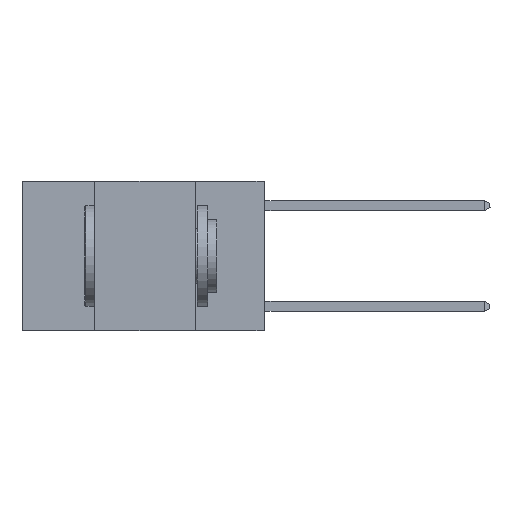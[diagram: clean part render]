
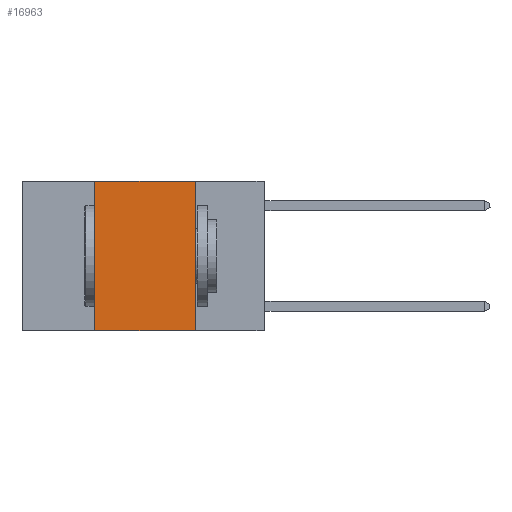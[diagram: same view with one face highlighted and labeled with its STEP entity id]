
A CAD part, left-side view. The second image highlights one B-rep face of the part: STEP entity #16963.
In plain terms, the highlighted planar face has unit normal (-1, 0, 0).
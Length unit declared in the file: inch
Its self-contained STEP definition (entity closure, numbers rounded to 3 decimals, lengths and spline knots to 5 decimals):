
#492 = CARTESIAN_POINT ( 'NONE',  ( 0., 0.42, 0. ) ) ;
#1504 = LINE ( 'NONE', #22077, #13023 ) ;
#2939 = VERTEX_POINT ( 'NONE', #27327 ) ;
#2967 = ORIENTED_EDGE ( 'NONE', *, *, #24986, .F. ) ;
#2998 = VECTOR ( 'NONE', #12646, 39.37008 ) ;
#4350 = PLANE ( 'NONE',  #23697 ) ;
#5289 = VERTEX_POINT ( 'NONE', #22720 ) ;
#6217 = LINE ( 'NONE', #11053, #22846 ) ;
#6974 = EDGE_CURVE ( 'NONE', #17826, #8032, #21175, .T. ) ;
#7304 = CARTESIAN_POINT ( 'NONE',  ( 0., 0.42, -0.37 ) ) ;
#8032 = VERTEX_POINT ( 'NONE', #492 ) ;
#8405 = ORIENTED_EDGE ( 'NONE', *, *, #6974, .F. ) ;
#8835 = DIRECTION ( 'NONE',  ( 0., -1., 0. ) ) ;
#9549 = CARTESIAN_POINT ( 'NONE',  ( 0., 0.17, 0. ) ) ;
#10318 = CARTESIAN_POINT ( 'NONE',  ( 0., 0.42, 0. ) ) ;
#11053 = CARTESIAN_POINT ( 'NONE',  ( 0., 0.6, 0. ) ) ;
#11268 = DIRECTION ( 'NONE',  ( 0., 0., -1. ) ) ;
#12646 = DIRECTION ( 'NONE',  ( 0., 0., 1. ) ) ;
#13023 = VECTOR ( 'NONE', #17570, 39.37008 ) ;
#13420 = EDGE_LOOP ( 'NONE', ( #14421, #2967, #8405, #14351 ) ) ;
#14351 = ORIENTED_EDGE ( 'NONE', *, *, #14888, .T. ) ;
#14421 = ORIENTED_EDGE ( 'NONE', *, *, #22596, .F. ) ;
#14888 = EDGE_CURVE ( 'NONE', #17826, #5289, #1504, .T. ) ;
#16352 = LINE ( 'NONE', #9549, #22328 ) ;
#16963 = ADVANCED_FACE ( 'NONE', ( #23442 ), #4350, .F. ) ;
#17570 = DIRECTION ( 'NONE',  ( 0., -1., 0. ) ) ;
#17826 = VERTEX_POINT ( 'NONE', #7304 ) ;
#20865 = DIRECTION ( 'NONE',  ( 0., 0., -1. ) ) ;
#21175 = LINE ( 'NONE', #10318, #2998 ) ;
#22077 = CARTESIAN_POINT ( 'NONE',  ( 0., 0.6, -0.37 ) ) ;
#22328 = VECTOR ( 'NONE', #20865, 39.37008 ) ;
#22495 = CARTESIAN_POINT ( 'NONE',  ( 0., 0.6, 0. ) ) ;
#22596 = EDGE_CURVE ( 'NONE', #2939, #5289, #16352, .T. ) ;
#22720 = CARTESIAN_POINT ( 'NONE',  ( 0., 0.17, -0.37 ) ) ;
#22846 = VECTOR ( 'NONE', #8835, 39.37008 ) ;
#23442 = FACE_OUTER_BOUND ( 'NONE', #13420, .T. ) ;
#23697 = AXIS2_PLACEMENT_3D ( 'NONE', #22495, #24701, #11268 ) ;
#24701 = DIRECTION ( 'NONE',  ( 1., 0., 0. ) ) ;
#24986 = EDGE_CURVE ( 'NONE', #8032, #2939, #6217, .T. ) ;
#27327 = CARTESIAN_POINT ( 'NONE',  ( 0., 0.17, 0. ) ) ;
